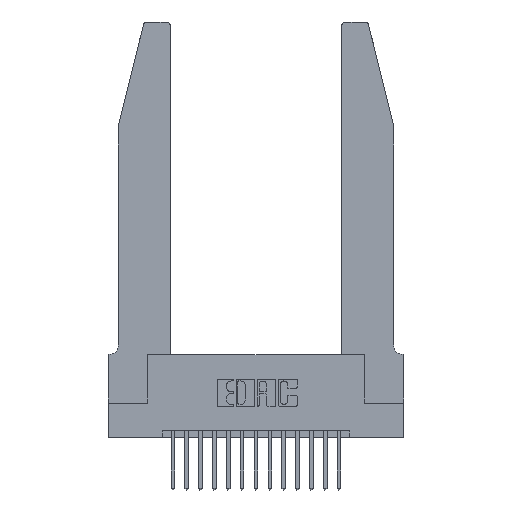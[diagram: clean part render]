
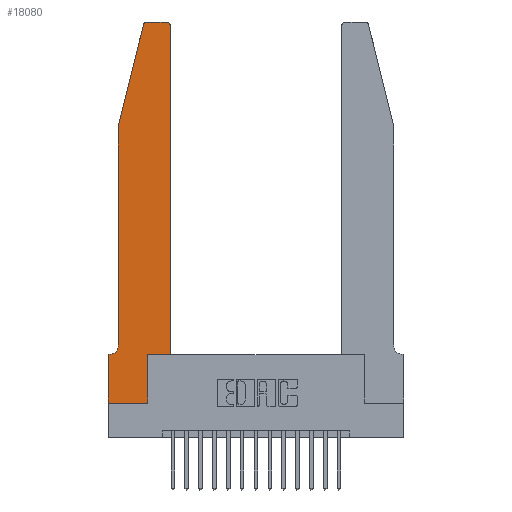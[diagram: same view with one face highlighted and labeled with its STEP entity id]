
A CAD part, top view. The second image highlights one B-rep face of the part: STEP entity #18080.
In plain terms, the highlighted planar face has unit normal (0, 0, 1).
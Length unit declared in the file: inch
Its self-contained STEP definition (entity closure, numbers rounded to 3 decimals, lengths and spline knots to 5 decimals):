
#176 = CARTESIAN_POINT ( 'NONE',  ( 0.0055, 0.35, 0.37 ) ) ;
#400 = DIRECTION ( 'NONE',  ( 0., 0., 1. ) ) ;
#452 = CARTESIAN_POINT ( 'NONE',  ( 0., 0.35, 0.37 ) ) ;
#609 = CARTESIAN_POINT ( 'NONE',  ( 0., 0., 0.37 ) ) ;
#632 = CARTESIAN_POINT ( 'NONE',  ( 0.284, 2.75, 0.37 ) ) ;
#975 = VERTEX_POINT ( 'NONE', #3234 ) ;
#997 = CARTESIAN_POINT ( 'NONE',  ( 0., 0., 0.37 ) ) ;
#1582 = CARTESIAN_POINT ( 'NONE',  ( 0.2865, 0.35, 0.37 ) ) ;
#1587 = LINE ( 'NONE', #13006, #8840 ) ;
#1684 = CARTESIAN_POINT ( 'NONE',  ( 0.2865, 0.35, 0.37 ) ) ;
#1836 = VERTEX_POINT ( 'NONE', #176 ) ;
#1922 = VECTOR ( 'NONE', #13440, 39.37008 ) ;
#2412 = CARTESIAN_POINT ( 'NONE',  ( 0.0055, 0.42, 0.37 ) ) ;
#2492 = LINE ( 'NONE', #6869, #14094 ) ;
#2541 = VERTEX_POINT ( 'NONE', #17579 ) ;
#2707 = ORIENTED_EDGE ( 'NONE', *, *, #16693, .T. ) ;
#2711 = CARTESIAN_POINT ( 'NONE',  ( 0.4505, 0.35, 0.37 ) ) ;
#2718 = EDGE_CURVE ( 'NONE', #3249, #975, #1587, .T. ) ;
#2830 = VECTOR ( 'NONE', #5697, 39.37008 ) ;
#2989 = DIRECTION ( 'NONE',  ( 1., 0., 0. ) ) ;
#3180 = EDGE_CURVE ( 'NONE', #14832, #6758, #15451, .T. ) ;
#3208 = ORIENTED_EDGE ( 'NONE', *, *, #16205, .T. ) ;
#3234 = CARTESIAN_POINT ( 'NONE',  ( 0.0755, 0.42, 0.37 ) ) ;
#3249 = VERTEX_POINT ( 'NONE', #14648 ) ;
#3372 = VECTOR ( 'NONE', #2989, 39.37008 ) ;
#3992 = ORIENTED_EDGE ( 'NONE', *, *, #12651, .T. ) ;
#4088 = EDGE_LOOP ( 'NONE', ( #11733, #18425, #2707, #7205, #3208, #3992, #18795, #11332, #17413, #6124, #5165, #9868 ) ) ;
#4222 = VECTOR ( 'NONE', #12073, 39.37008 ) ;
#4308 = VECTOR ( 'NONE', #12601, 39.37008 ) ;
#4480 = CARTESIAN_POINT ( 'NONE',  ( 0.4505, 2.72, 0.37 ) ) ;
#4725 = DIRECTION ( 'NONE',  ( 1., 0., 0. ) ) ;
#4866 = VECTOR ( 'NONE', #14238, 39.37008 ) ;
#5165 = ORIENTED_EDGE ( 'NONE', *, *, #6237, .T. ) ;
#5205 = DIRECTION ( 'NONE',  ( -1., 0., 0. ) ) ;
#5673 = LINE ( 'NONE', #997, #4308 ) ;
#5697 = DIRECTION ( 'NONE',  ( 0., 1., 0. ) ) ;
#6033 = LINE ( 'NONE', #1684, #4222 ) ;
#6124 = ORIENTED_EDGE ( 'NONE', *, *, #3180, .T. ) ;
#6223 = PLANE ( 'NONE',  #13272 ) ;
#6237 = EDGE_CURVE ( 'NONE', #6758, #17379, #8276, .T. ) ;
#6361 = EDGE_CURVE ( 'NONE', #14520, #18754, #11242, .T. ) ;
#6572 = EDGE_CURVE ( 'NONE', #8428, #14166, #7158, .T. ) ;
#6758 = VERTEX_POINT ( 'NONE', #16732 ) ;
#6860 = AXIS2_PLACEMENT_3D ( 'NONE', #10464, #400, #4725 ) ;
#6869 = CARTESIAN_POINT ( 'NONE',  ( 0.0755, 0.35, 0.37 ) ) ;
#6958 = AXIS2_PLACEMENT_3D ( 'NONE', #14064, #12407, #13875 ) ;
#7158 = LINE ( 'NONE', #609, #1922 ) ;
#7166 = VECTOR ( 'NONE', #13631, 39.37008 ) ;
#7205 = ORIENTED_EDGE ( 'NONE', *, *, #2718, .T. ) ;
#7619 = EDGE_CURVE ( 'NONE', #17379, #14520, #14170, .T. ) ;
#7810 = CARTESIAN_POINT ( 'NONE',  ( 0., 0.35, 0.37 ) ) ;
#8276 = LINE ( 'NONE', #2711, #2830 ) ;
#8428 = VERTEX_POINT ( 'NONE', #7810 ) ;
#8701 = FACE_OUTER_BOUND ( 'NONE', #4088, .T. ) ;
#8840 = VECTOR ( 'NONE', #14564, 39.37008 ) ;
#9562 = EDGE_CURVE ( 'NONE', #18754, #15511, #11957, .T. ) ;
#9868 = ORIENTED_EDGE ( 'NONE', *, *, #7619, .T. ) ;
#10351 = AXIS2_PLACEMENT_3D ( 'NONE', #2412, #15214, #5205 ) ;
#10464 = CARTESIAN_POINT ( 'NONE',  ( 0.284, 2.72, 0.37 ) ) ;
#11185 = DIRECTION ( 'NONE',  ( -1., 0., 0. ) ) ;
#11242 = LINE ( 'NONE', #12876, #4866 ) ;
#11332 = ORIENTED_EDGE ( 'NONE', *, *, #12331, .T. ) ;
#11638 = CARTESIAN_POINT ( 'NONE',  ( 0.25487, 2.72718, 0.37 ) ) ;
#11733 = ORIENTED_EDGE ( 'NONE', *, *, #6361, .T. ) ;
#11957 = CIRCLE ( 'NONE', #6860, 0.03 ) ;
#12073 = DIRECTION ( 'NONE',  ( 0., 1., 0. ) ) ;
#12076 = DIRECTION ( 'NONE',  ( 1., 0., 0. ) ) ;
#12331 = EDGE_CURVE ( 'NONE', #14166, #2541, #5673, .T. ) ;
#12407 = DIRECTION ( 'NONE',  ( 0., 0., 1. ) ) ;
#12601 = DIRECTION ( 'NONE',  ( 1., 0., 0. ) ) ;
#12651 = EDGE_CURVE ( 'NONE', #1836, #8428, #2492, .T. ) ;
#12876 = CARTESIAN_POINT ( 'NONE',  ( 0.2605, 2.75, 0.37 ) ) ;
#13006 = CARTESIAN_POINT ( 'NONE',  ( 0.0755, 2., 0.37 ) ) ;
#13272 = AXIS2_PLACEMENT_3D ( 'NONE', #452, #15081, #12076 ) ;
#13440 = DIRECTION ( 'NONE',  ( 0., -1., 0. ) ) ;
#13631 = DIRECTION ( 'NONE',  ( -0.239, -0.971, 0. ) ) ;
#13875 = DIRECTION ( 'NONE',  ( 1., 0., 0. ) ) ;
#14064 = CARTESIAN_POINT ( 'NONE',  ( 0.4205, 2.72, 0.37 ) ) ;
#14094 = VECTOR ( 'NONE', #11185, 39.37008 ) ;
#14166 = VERTEX_POINT ( 'NONE', #18717 ) ;
#14170 = CIRCLE ( 'NONE', #6958, 0.03 ) ;
#14238 = DIRECTION ( 'NONE',  ( -1., 0., 0. ) ) ;
#14520 = VERTEX_POINT ( 'NONE', #15544 ) ;
#14564 = DIRECTION ( 'NONE',  ( 0., -1., 0. ) ) ;
#14648 = CARTESIAN_POINT ( 'NONE',  ( 0.0755, 2., 0.37 ) ) ;
#14832 = VERTEX_POINT ( 'NONE', #1582 ) ;
#15081 = DIRECTION ( 'NONE',  ( 0., 0., 1. ) ) ;
#15118 = CIRCLE ( 'NONE', #10351, 0.07 ) ;
#15214 = DIRECTION ( 'NONE',  ( 0., 0., -1. ) ) ;
#15451 = LINE ( 'NONE', #17578, #3372 ) ;
#15511 = VERTEX_POINT ( 'NONE', #11638 ) ;
#15543 = EDGE_CURVE ( 'NONE', #2541, #14832, #6033, .T. ) ;
#15544 = CARTESIAN_POINT ( 'NONE',  ( 0.4205, 2.75, 0.37 ) ) ;
#16205 = EDGE_CURVE ( 'NONE', #975, #1836, #15118, .T. ) ;
#16693 = EDGE_CURVE ( 'NONE', #15511, #3249, #18615, .T. ) ;
#16732 = CARTESIAN_POINT ( 'NONE',  ( 0.4505, 0.35, 0.37 ) ) ;
#17379 = VERTEX_POINT ( 'NONE', #4480 ) ;
#17413 = ORIENTED_EDGE ( 'NONE', *, *, #15543, .T. ) ;
#17578 = CARTESIAN_POINT ( 'NONE',  ( 0.4505, 0.35, 0.37 ) ) ;
#17579 = CARTESIAN_POINT ( 'NONE',  ( 0.2865, 0., 0.37 ) ) ;
#17995 = CARTESIAN_POINT ( 'NONE',  ( 0.0755, 2., 0.37 ) ) ;
#18080 = ADVANCED_FACE ( 'NONE', ( #8701 ), #6223, .T. ) ;
#18425 = ORIENTED_EDGE ( 'NONE', *, *, #9562, .T. ) ;
#18615 = LINE ( 'NONE', #17995, #7166 ) ;
#18717 = CARTESIAN_POINT ( 'NONE',  ( 0., 0., 0.37 ) ) ;
#18754 = VERTEX_POINT ( 'NONE', #632 ) ;
#18795 = ORIENTED_EDGE ( 'NONE', *, *, #6572, .T. ) ;
